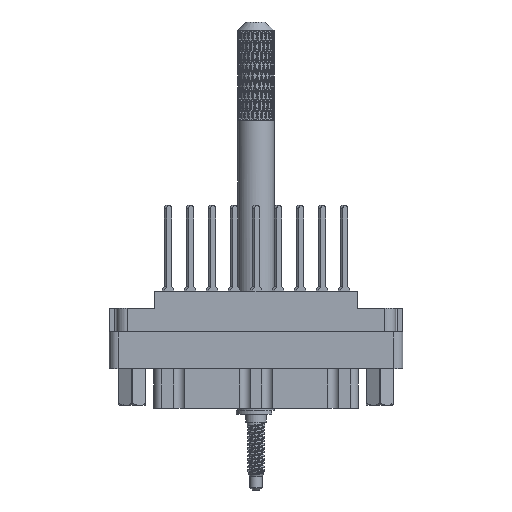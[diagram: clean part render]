
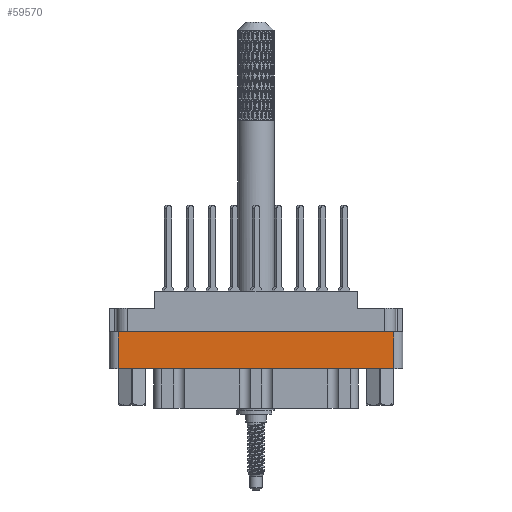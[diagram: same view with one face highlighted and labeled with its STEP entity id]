
A CAD part, front view. The second image highlights one B-rep face of the part: STEP entity #59570.
In plain terms, the highlighted planar face has unit normal (0, -1, 0).
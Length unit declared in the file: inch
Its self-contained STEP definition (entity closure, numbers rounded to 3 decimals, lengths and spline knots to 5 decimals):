
#639 = CARTESIAN_POINT ( 'NONE',  ( -0.938, -0.438, -0.798 ) ) ;
#1921 = CARTESIAN_POINT ( 'NONE',  ( -1., -0.438, -0.277 ) ) ;
#4504 = CARTESIAN_POINT ( 'NONE',  ( 0.938, -0.438, -0.529 ) ) ;
#9723 = CARTESIAN_POINT ( 'NONE',  ( -0.938, -0.438, -0.529 ) ) ;
#17744 = VERTEX_POINT ( 'NONE', #33568 ) ;
#18354 = DIRECTION ( 'NONE',  ( 0., 0., -1. ) ) ;
#24066 = EDGE_CURVE ( 'NONE', #26991, #33338, #44505, .T. ) ;
#26746 = CARTESIAN_POINT ( 'NONE',  ( -0.938, -0.438, -0.798 ) ) ;
#26991 = VERTEX_POINT ( 'NONE', #45951 ) ;
#27667 = DIRECTION ( 'NONE',  ( 1., 0., 0. ) ) ;
#28228 = EDGE_LOOP ( 'NONE', ( #28698, #32168, #53649, #44153 ) ) ;
#28698 = ORIENTED_EDGE ( 'NONE', *, *, #35962, .F. ) ;
#29268 = VECTOR ( 'NONE', #27667, 39.37008 ) ;
#29643 = EDGE_CURVE ( 'NONE', #17744, #38065, #100876, .T. ) ;
#32168 = ORIENTED_EDGE ( 'NONE', *, *, #29643, .F. ) ;
#32618 = AXIS2_PLACEMENT_3D ( 'NONE', #26746, #95159, #18354 ) ;
#33338 = VERTEX_POINT ( 'NONE', #41843 ) ;
#33568 = CARTESIAN_POINT ( 'NONE',  ( 0.938, -0.438, -0.529 ) ) ;
#34255 = DIRECTION ( 'NONE',  ( 0., 0., 1. ) ) ;
#34395 = VECTOR ( 'NONE', #90797, 39.37008 ) ;
#35962 = EDGE_CURVE ( 'NONE', #38065, #26991, #77409, .T. ) ;
#36892 = LINE ( 'NONE', #78965, #68185 ) ;
#38065 = VERTEX_POINT ( 'NONE', #9723 ) ;
#41843 = CARTESIAN_POINT ( 'NONE',  ( 0.938, -0.438, -0.277 ) ) ;
#42089 = EDGE_CURVE ( 'NONE', #17744, #33338, #36892, .T. ) ;
#44153 = ORIENTED_EDGE ( 'NONE', *, *, #24066, .F. ) ;
#44505 = LINE ( 'NONE', #1921, #29268 ) ;
#45869 = DIRECTION ( 'NONE',  ( 0., 0., 1. ) ) ;
#45951 = CARTESIAN_POINT ( 'NONE',  ( -0.938, -0.438, -0.277 ) ) ;
#52020 = FACE_OUTER_BOUND ( 'NONE', #28228, .T. ) ;
#53649 = ORIENTED_EDGE ( 'NONE', *, *, #42089, .T. ) ;
#59570 = ADVANCED_FACE ( 'NONE', ( #52020 ), #103578, .T. ) ;
#62317 = VECTOR ( 'NONE', #34255, 39.37008 ) ;
#68185 = VECTOR ( 'NONE', #45869, 39.37008 ) ;
#77409 = LINE ( 'NONE', #639, #62317 ) ;
#78965 = CARTESIAN_POINT ( 'NONE',  ( 0.938, -0.438, -0.798 ) ) ;
#90797 = DIRECTION ( 'NONE',  ( -1., 0., 0. ) ) ;
#95159 = DIRECTION ( 'NONE',  ( 0., -1., 0. ) ) ;
#100876 = LINE ( 'NONE', #4504, #34395 ) ;
#103578 = PLANE ( 'NONE',  #32618 ) ;
